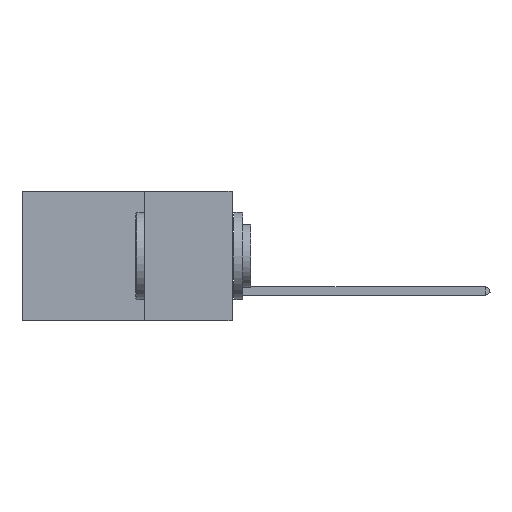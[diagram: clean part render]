
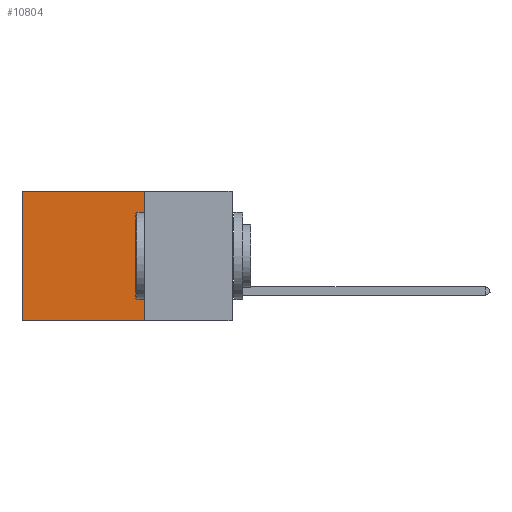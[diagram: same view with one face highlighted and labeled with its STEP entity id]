
A CAD part, left-side view. The second image highlights one B-rep face of the part: STEP entity #10804.
In plain terms, the highlighted planar face has unit normal (-1, 0, 0).
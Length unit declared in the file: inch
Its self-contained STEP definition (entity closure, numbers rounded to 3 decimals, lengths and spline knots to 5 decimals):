
#152 = VECTOR ( 'NONE', #8918, 39.37008 ) ;
#351 = CARTESIAN_POINT ( 'NONE',  ( 0.2875, 0.25, -0.37 ) ) ;
#474 = ORIENTED_EDGE ( 'NONE', *, *, #20635, .F. ) ;
#507 = CARTESIAN_POINT ( 'NONE',  ( 0.2875, 0.6, 0. ) ) ;
#1026 = LINE ( 'NONE', #18598, #19023 ) ;
#1564 = DIRECTION ( 'NONE',  ( 0., 0., -1. ) ) ;
#1750 = ORIENTED_EDGE ( 'NONE', *, *, #19148, .T. ) ;
#1789 = DIRECTION ( 'NONE',  ( 0., 0., -1. ) ) ;
#2318 = AXIS2_PLACEMENT_3D ( 'NONE', #12963, #16433, #1789 ) ;
#2376 = ORIENTED_EDGE ( 'NONE', *, *, #18738, .F. ) ;
#3225 = CARTESIAN_POINT ( 'NONE',  ( 0.2875, 0.25, 0. ) ) ;
#3478 = PLANE ( 'NONE',  #2318 ) ;
#3783 = EDGE_CURVE ( 'NONE', #7342, #14526, #1026, .T. ) ;
#6063 = CARTESIAN_POINT ( 'NONE',  ( 0.2875, 0.25, 0. ) ) ;
#7342 = VERTEX_POINT ( 'NONE', #507 ) ;
#7874 = VECTOR ( 'NONE', #20059, 39.37008 ) ;
#8574 = LINE ( 'NONE', #6063, #19851 ) ;
#8918 = DIRECTION ( 'NONE',  ( 0., 1., 0. ) ) ;
#10804 = ADVANCED_FACE ( 'NONE', ( #19693 ), #3478, .F. ) ;
#11040 = LINE ( 'NONE', #13396, #7874 ) ;
#12963 = CARTESIAN_POINT ( 'NONE',  ( 0.2875, 0.25, 0. ) ) ;
#13396 = CARTESIAN_POINT ( 'NONE',  ( 0.2875, 0.25, 0. ) ) ;
#14526 = VERTEX_POINT ( 'NONE', #19080 ) ;
#16316 = VERTEX_POINT ( 'NONE', #351 ) ;
#16433 = DIRECTION ( 'NONE',  ( 1., 0., 0. ) ) ;
#17342 = CARTESIAN_POINT ( 'NONE',  ( 0.2875, 0.25, -0.37 ) ) ;
#17620 = LINE ( 'NONE', #17342, #152 ) ;
#18369 = DIRECTION ( 'NONE',  ( 0., 0., -1. ) ) ;
#18381 = ORIENTED_EDGE ( 'NONE', *, *, #3783, .T. ) ;
#18471 = VERTEX_POINT ( 'NONE', #3225 ) ;
#18598 = CARTESIAN_POINT ( 'NONE',  ( 0.2875, 0.6, 0. ) ) ;
#18738 = EDGE_CURVE ( 'NONE', #16316, #14526, #17620, .T. ) ;
#19023 = VECTOR ( 'NONE', #18369, 39.37008 ) ;
#19080 = CARTESIAN_POINT ( 'NONE',  ( 0.2875, 0.6, -0.37 ) ) ;
#19148 = EDGE_CURVE ( 'NONE', #18471, #7342, #11040, .T. ) ;
#19693 = FACE_OUTER_BOUND ( 'NONE', #20244, .T. ) ;
#19851 = VECTOR ( 'NONE', #1564, 39.37008 ) ;
#20059 = DIRECTION ( 'NONE',  ( 0., 1., 0. ) ) ;
#20244 = EDGE_LOOP ( 'NONE', ( #18381, #2376, #474, #1750 ) ) ;
#20635 = EDGE_CURVE ( 'NONE', #18471, #16316, #8574, .T. ) ;
